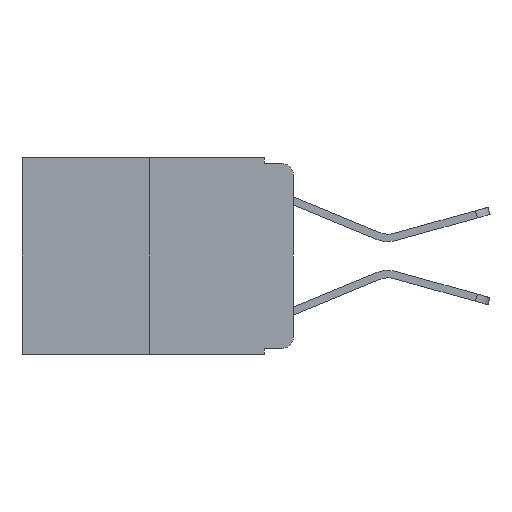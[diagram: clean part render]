
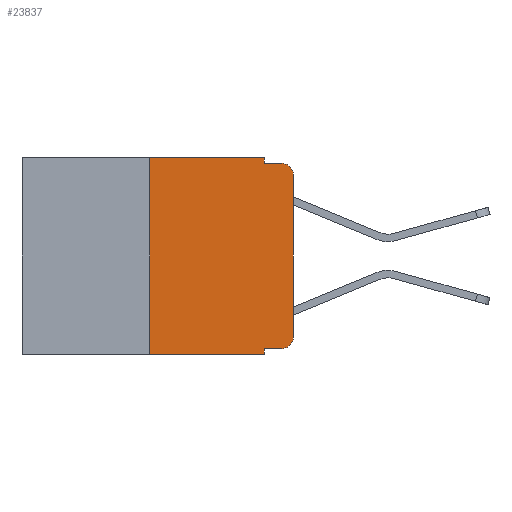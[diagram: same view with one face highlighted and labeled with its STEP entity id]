
A CAD part, left-side view. The second image highlights one B-rep face of the part: STEP entity #23837.
In plain terms, the highlighted planar face has unit normal (-1, 0, 0).
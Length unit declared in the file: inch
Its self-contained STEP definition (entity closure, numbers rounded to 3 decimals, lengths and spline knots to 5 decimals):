
#162 = ORIENTED_EDGE ( 'NONE', *, *, #15352, .F. ) ;
#275 = VECTOR ( 'NONE', #15872, 39.37008 ) ;
#308 = FACE_OUTER_BOUND ( 'NONE', #1106, .T. ) ;
#767 = CARTESIAN_POINT ( 'NONE',  ( 0., 0.02, -0.333 ) ) ;
#930 = LINE ( 'NONE', #16186, #23394 ) ;
#1106 = EDGE_LOOP ( 'NONE', ( #8205, #6759, #6154, #4380, #17682, #162, #11480, #10698, #20771, #23345 ) ) ;
#1138 = EDGE_CURVE ( 'NONE', #18104, #6477, #4110, .T. ) ;
#1593 = CARTESIAN_POINT ( 'NONE',  ( 0., 0.25, -0.343 ) ) ;
#2256 = CARTESIAN_POINT ( 'NONE',  ( 0., 0.051, -0.333 ) ) ;
#2268 = EDGE_CURVE ( 'NONE', #18995, #6477, #5277, .T. ) ;
#2368 = CARTESIAN_POINT ( 'NONE',  ( 0., 0., -0.03 ) ) ;
#2790 = VECTOR ( 'NONE', #19906, 39.37008 ) ;
#3634 = VECTOR ( 'NONE', #9043, 39.37008 ) ;
#4033 = VERTEX_POINT ( 'NONE', #7823 ) ;
#4104 = CARTESIAN_POINT ( 'NONE',  ( 0., 0.051, 0. ) ) ;
#4110 = LINE ( 'NONE', #12014, #275 ) ;
#4134 = DIRECTION ( 'NONE',  ( 1., 0., 0. ) ) ;
#4380 = ORIENTED_EDGE ( 'NONE', *, *, #8807, .F. ) ;
#5277 = CIRCLE ( 'NONE', #16028, 0.02 ) ;
#5991 = LINE ( 'NONE', #8891, #3634 ) ;
#6154 = ORIENTED_EDGE ( 'NONE', *, *, #1138, .F. ) ;
#6376 = EDGE_CURVE ( 'NONE', #6810, #18995, #5991, .T. ) ;
#6477 = VERTEX_POINT ( 'NONE', #18686 ) ;
#6666 = CIRCLE ( 'NONE', #19492, 0.02 ) ;
#6759 = ORIENTED_EDGE ( 'NONE', *, *, #2268, .T. ) ;
#6775 = DIRECTION ( 'NONE',  ( 0., 0., -1. ) ) ;
#6810 = VERTEX_POINT ( 'NONE', #19651 ) ;
#7823 = CARTESIAN_POINT ( 'NONE',  ( 0., 0.25, 0. ) ) ;
#7849 = VECTOR ( 'NONE', #17762, 39.37008 ) ;
#7857 = CARTESIAN_POINT ( 'NONE',  ( 0., 0.02, -0.313 ) ) ;
#8205 = ORIENTED_EDGE ( 'NONE', *, *, #6376, .T. ) ;
#8420 = LINE ( 'NONE', #10266, #2790 ) ;
#8807 = EDGE_CURVE ( 'NONE', #11384, #18104, #19214, .T. ) ;
#8891 = CARTESIAN_POINT ( 'NONE',  ( 0., 0., 0. ) ) ;
#9043 = DIRECTION ( 'NONE',  ( 0., 0., 1. ) ) ;
#9185 = VECTOR ( 'NONE', #10436, 39.37008 ) ;
#10266 = CARTESIAN_POINT ( 'NONE',  ( 0., 0.25, 0. ) ) ;
#10436 = DIRECTION ( 'NONE',  ( 0., 0., -1. ) ) ;
#10501 = DIRECTION ( 'NONE',  ( -1., 0., 0. ) ) ;
#10698 = ORIENTED_EDGE ( 'NONE', *, *, #13712, .F. ) ;
#11384 = VERTEX_POINT ( 'NONE', #4104 ) ;
#11445 = LINE ( 'NONE', #14841, #16169 ) ;
#11480 = ORIENTED_EDGE ( 'NONE', *, *, #15351, .T. ) ;
#11516 = CARTESIAN_POINT ( 'NONE',  ( 0., 0.473, 0. ) ) ;
#11589 = DIRECTION ( 'NONE',  ( 0., 0., -1. ) ) ;
#12014 = CARTESIAN_POINT ( 'NONE',  ( 0., 0.051, -0.01 ) ) ;
#12469 = AXIS2_PLACEMENT_3D ( 'NONE', #11516, #4134, #11589 ) ;
#12769 = VERTEX_POINT ( 'NONE', #767 ) ;
#13151 = LINE ( 'NONE', #2256, #19911 ) ;
#13160 = DIRECTION ( 'NONE',  ( 0., 0., -1. ) ) ;
#13448 = LINE ( 'NONE', #17839, #7849 ) ;
#13712 = EDGE_CURVE ( 'NONE', #20502, #13805, #11445, .T. ) ;
#13805 = VERTEX_POINT ( 'NONE', #22690 ) ;
#14286 = EDGE_CURVE ( 'NONE', #12769, #6810, #6666, .T. ) ;
#14841 = CARTESIAN_POINT ( 'NONE',  ( 0., 0.051, 0. ) ) ;
#15194 = EDGE_CURVE ( 'NONE', #20502, #12769, #13151, .T. ) ;
#15198 = PLANE ( 'NONE',  #12469 ) ;
#15351 = EDGE_CURVE ( 'NONE', #23146, #13805, #13448, .T. ) ;
#15352 = EDGE_CURVE ( 'NONE', #23146, #4033, #8420, .T. ) ;
#15872 = DIRECTION ( 'NONE',  ( 0., -1., 0. ) ) ;
#16028 = AXIS2_PLACEMENT_3D ( 'NONE', #16249, #10501, #6775 ) ;
#16169 = VECTOR ( 'NONE', #13160, 39.37008 ) ;
#16186 = CARTESIAN_POINT ( 'NONE',  ( 0., 0.473, 0. ) ) ;
#16249 = CARTESIAN_POINT ( 'NONE',  ( 0., 0.02, -0.03 ) ) ;
#17386 = EDGE_CURVE ( 'NONE', #4033, #11384, #930, .T. ) ;
#17682 = ORIENTED_EDGE ( 'NONE', *, *, #17386, .F. ) ;
#17762 = DIRECTION ( 'NONE',  ( 0., -1., 0. ) ) ;
#17839 = CARTESIAN_POINT ( 'NONE',  ( 0., 0.473, -0.343 ) ) ;
#18104 = VERTEX_POINT ( 'NONE', #18267 ) ;
#18267 = CARTESIAN_POINT ( 'NONE',  ( 0., 0.051, -0.01 ) ) ;
#18686 = CARTESIAN_POINT ( 'NONE',  ( 0., 0.02, -0.01 ) ) ;
#18995 = VERTEX_POINT ( 'NONE', #2368 ) ;
#19212 = DIRECTION ( 'NONE',  ( -1., 0., 0. ) ) ;
#19214 = LINE ( 'NONE', #21879, #9185 ) ;
#19492 = AXIS2_PLACEMENT_3D ( 'NONE', #7857, #19212, #21091 ) ;
#19651 = CARTESIAN_POINT ( 'NONE',  ( 0., 0., -0.313 ) ) ;
#19906 = DIRECTION ( 'NONE',  ( 0., 0., 1. ) ) ;
#19911 = VECTOR ( 'NONE', #21309, 39.37008 ) ;
#20502 = VERTEX_POINT ( 'NONE', #23513 ) ;
#20771 = ORIENTED_EDGE ( 'NONE', *, *, #15194, .T. ) ;
#21091 = DIRECTION ( 'NONE',  ( 0., 0., -1. ) ) ;
#21309 = DIRECTION ( 'NONE',  ( 0., -1., 0. ) ) ;
#21879 = CARTESIAN_POINT ( 'NONE',  ( 0., 0.051, 0. ) ) ;
#22047 = DIRECTION ( 'NONE',  ( 0., -1., 0. ) ) ;
#22690 = CARTESIAN_POINT ( 'NONE',  ( 0., 0.051, -0.343 ) ) ;
#23146 = VERTEX_POINT ( 'NONE', #1593 ) ;
#23345 = ORIENTED_EDGE ( 'NONE', *, *, #14286, .T. ) ;
#23394 = VECTOR ( 'NONE', #22047, 39.37008 ) ;
#23513 = CARTESIAN_POINT ( 'NONE',  ( 0., 0.051, -0.333 ) ) ;
#23837 = ADVANCED_FACE ( 'NONE', ( #308 ), #15198, .F. ) ;
